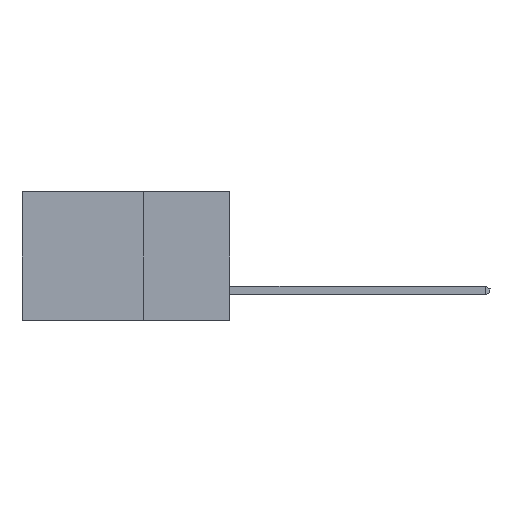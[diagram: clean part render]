
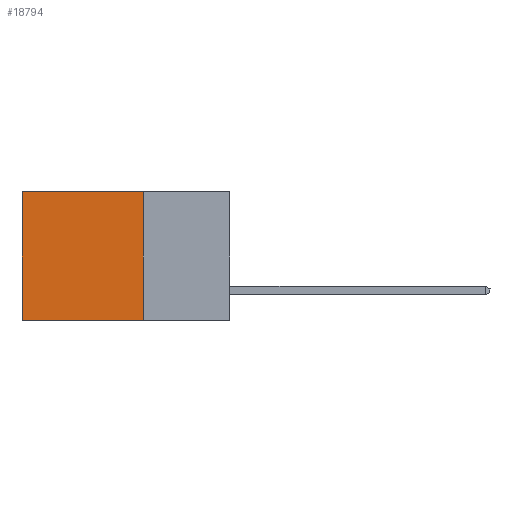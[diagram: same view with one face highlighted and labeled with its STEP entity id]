
A CAD part, left-side view. The second image highlights one B-rep face of the part: STEP entity #18794.
In plain terms, the highlighted planar face has unit normal (-1, 0, 0).
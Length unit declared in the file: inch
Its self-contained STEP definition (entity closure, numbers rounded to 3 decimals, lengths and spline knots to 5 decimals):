
#1071 = CARTESIAN_POINT ( 'NONE',  ( 0.2615, 0.25, -0.37 ) ) ;
#3412 = CARTESIAN_POINT ( 'NONE',  ( 0.2615, 0.25, -0.37 ) ) ;
#5219 = ORIENTED_EDGE ( 'NONE', *, *, #14415, .T. ) ;
#5616 = ORIENTED_EDGE ( 'NONE', *, *, #12538, .F. ) ;
#6011 = AXIS2_PLACEMENT_3D ( 'NONE', #3412, #11269, #19572 ) ;
#8122 = DIRECTION ( 'NONE',  ( 0., 1., 0. ) ) ;
#9034 = CARTESIAN_POINT ( 'NONE',  ( 0.2615, 0.25, 0. ) ) ;
#9363 = PLANE ( 'NONE',  #6011 ) ;
#10135 = VECTOR ( 'NONE', #16178, 39.37008 ) ;
#10231 = CARTESIAN_POINT ( 'NONE',  ( 0.2615, 0.6, -0.37 ) ) ;
#11011 = VERTEX_POINT ( 'NONE', #18655 ) ;
#11040 = EDGE_LOOP ( 'NONE', ( #17791, #19407, #5616, #5219 ) ) ;
#11187 = VECTOR ( 'NONE', #8122, 39.37008 ) ;
#11269 = DIRECTION ( 'NONE',  ( 1., 0., 0. ) ) ;
#11363 = CARTESIAN_POINT ( 'NONE',  ( 0.2615, 0.25, -0.37 ) ) ;
#11434 = VECTOR ( 'NONE', #13049, 39.37008 ) ;
#12538 = EDGE_CURVE ( 'NONE', #19468, #13757, #17094, .T. ) ;
#13049 = DIRECTION ( 'NONE',  ( 0., 0., -1. ) ) ;
#13222 = FACE_OUTER_BOUND ( 'NONE', #11040, .T. ) ;
#13757 = VERTEX_POINT ( 'NONE', #1071 ) ;
#13860 = CARTESIAN_POINT ( 'NONE',  ( 0.2615, 0.25, -0.37 ) ) ;
#14415 = EDGE_CURVE ( 'NONE', #19468, #11011, #17588, .T. ) ;
#16178 = DIRECTION ( 'NONE',  ( 0., 1., 0. ) ) ;
#16668 = DIRECTION ( 'NONE',  ( 0., 0., -1. ) ) ;
#17094 = LINE ( 'NONE', #11363, #11434 ) ;
#17588 = LINE ( 'NONE', #23776, #11187 ) ;
#17791 = ORIENTED_EDGE ( 'NONE', *, *, #19495, .T. ) ;
#18581 = CARTESIAN_POINT ( 'NONE',  ( 0.2615, 0.6, -0.37 ) ) ;
#18655 = CARTESIAN_POINT ( 'NONE',  ( 0.2615, 0.6, 0. ) ) ;
#18794 = ADVANCED_FACE ( 'NONE', ( #13222 ), #9363, .F. ) ;
#18947 = EDGE_CURVE ( 'NONE', #13757, #24661, #21859, .T. ) ;
#19407 = ORIENTED_EDGE ( 'NONE', *, *, #18947, .F. ) ;
#19468 = VERTEX_POINT ( 'NONE', #9034 ) ;
#19495 = EDGE_CURVE ( 'NONE', #11011, #24661, #22582, .T. ) ;
#19572 = DIRECTION ( 'NONE',  ( 0., 0., -1. ) ) ;
#19655 = VECTOR ( 'NONE', #16668, 39.37008 ) ;
#21859 = LINE ( 'NONE', #13860, #10135 ) ;
#22582 = LINE ( 'NONE', #18581, #19655 ) ;
#23776 = CARTESIAN_POINT ( 'NONE',  ( 0.2615, 0.25, 0. ) ) ;
#24661 = VERTEX_POINT ( 'NONE', #10231 ) ;
